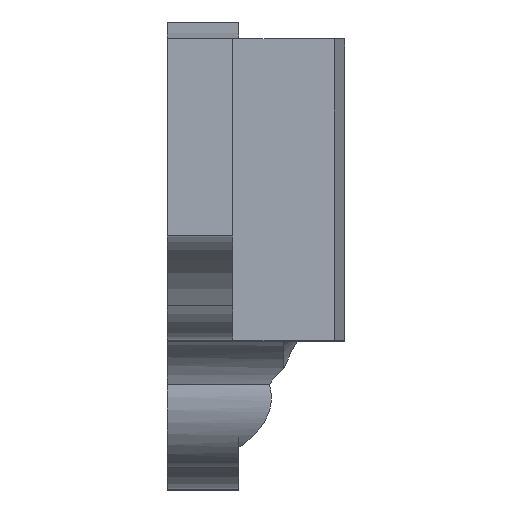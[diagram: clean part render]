
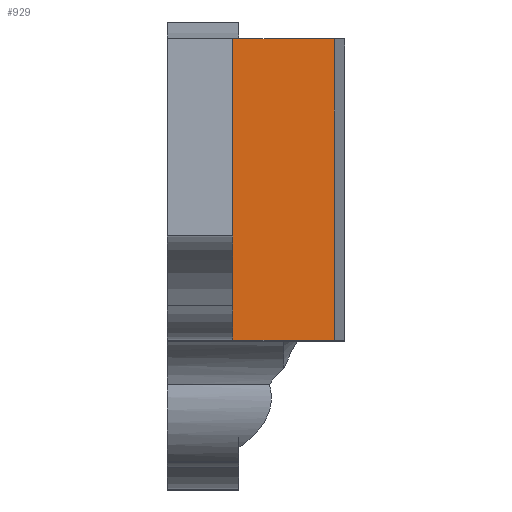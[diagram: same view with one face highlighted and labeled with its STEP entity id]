
A CAD part, top view. The second image highlights one B-rep face of the part: STEP entity #929.
In plain terms, the highlighted planar face has unit normal (0, 0, 1).
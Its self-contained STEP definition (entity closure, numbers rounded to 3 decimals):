
#114 = DIRECTION ( 'NONE',  ( 0., 1., 0. ) ) ;
#142 = DIRECTION ( 'NONE',  ( 1., 0., 0. ) ) ;
#168 = VERTEX_POINT ( 'NONE', #263 ) ;
#223 = VECTOR ( 'NONE', #1184, 1000. ) ;
#230 = CARTESIAN_POINT ( 'NONE',  ( 20.69, -8.425, 114.976 ) ) ;
#263 = CARTESIAN_POINT ( 'NONE',  ( 15.17, -8.425, 114.976 ) ) ;
#327 = VERTEX_POINT ( 'NONE', #1134 ) ;
#340 = EDGE_CURVE ( 'NONE', #168, #512, #1031, .T. ) ;
#363 = PLANE ( 'NONE',  #1123 ) ;
#364 = VERTEX_POINT ( 'NONE', #388 ) ;
#379 = VECTOR ( 'NONE', #114, 1000. ) ;
#388 = CARTESIAN_POINT ( 'NONE',  ( 20.188, -8.425, 114.976 ) ) ;
#426 = ORIENTED_EDGE ( 'NONE', *, *, #1178, .T. ) ;
#512 = VERTEX_POINT ( 'NONE', #1059 ) ;
#595 = VECTOR ( 'NONE', #1244, 1000. ) ;
#639 = CARTESIAN_POINT ( 'NONE',  ( 20.188, -26.534, 114.976 ) ) ;
#660 = CARTESIAN_POINT ( 'NONE',  ( 20.69, -2.905, 114.976 ) ) ;
#679 = FACE_OUTER_BOUND ( 'NONE', #996, .T. ) ;
#764 = CARTESIAN_POINT ( 'NONE',  ( 37.28, -23.305, 114.976 ) ) ;
#876 = DIRECTION ( 'NONE',  ( 0., 0., 1. ) ) ;
#905 = ORIENTED_EDGE ( 'NONE', *, *, #1004, .F. ) ;
#924 = ORIENTED_EDGE ( 'NONE', *, *, #1362, .F. ) ;
#929 = ADVANCED_FACE ( 'NONE', ( #679 ), #363, .T. ) ;
#952 = LINE ( 'NONE', #639, #379 ) ;
#996 = EDGE_LOOP ( 'NONE', ( #924, #426, #905, #1029 ) ) ;
#1004 = EDGE_CURVE ( 'NONE', #168, #364, #1177, .T. ) ;
#1029 = ORIENTED_EDGE ( 'NONE', *, *, #340, .T. ) ;
#1031 = LINE ( 'NONE', #1324, #595 ) ;
#1059 = CARTESIAN_POINT ( 'NONE',  ( 15.17, -23.305, 114.976 ) ) ;
#1103 = LINE ( 'NONE', #764, #1336 ) ;
#1123 = AXIS2_PLACEMENT_3D ( 'NONE', #660, #876, #142 ) ;
#1134 = CARTESIAN_POINT ( 'NONE',  ( 20.188, -23.305, 114.976 ) ) ;
#1177 = LINE ( 'NONE', #230, #223 ) ;
#1178 = EDGE_CURVE ( 'NONE', #327, #364, #952, .T. ) ;
#1184 = DIRECTION ( 'NONE',  ( 1., 0., 0. ) ) ;
#1244 = DIRECTION ( 'NONE',  ( 0., -1., 0. ) ) ;
#1306 = DIRECTION ( 'NONE',  ( -1., 0., 0. ) ) ;
#1324 = CARTESIAN_POINT ( 'NONE',  ( 15.17, -2.905, 114.976 ) ) ;
#1336 = VECTOR ( 'NONE', #1306, 1000. ) ;
#1362 = EDGE_CURVE ( 'NONE', #327, #512, #1103, .T. ) ;
